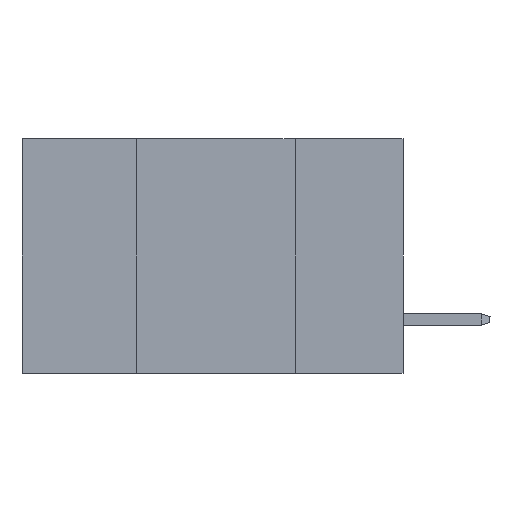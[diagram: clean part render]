
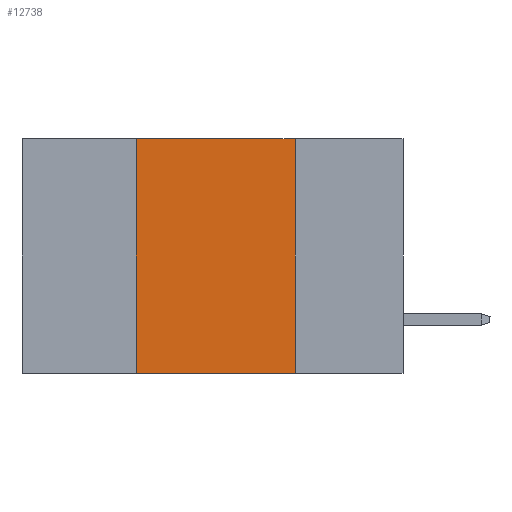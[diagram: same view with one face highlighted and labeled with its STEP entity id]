
A CAD part, left-side view. The second image highlights one B-rep face of the part: STEP entity #12738.
In plain terms, the highlighted planar face has unit normal (-1, 0, 0).
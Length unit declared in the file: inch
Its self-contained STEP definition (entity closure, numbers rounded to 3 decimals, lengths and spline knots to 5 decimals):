
#329 = CARTESIAN_POINT ( 'NONE',  ( 0., 0.17, 0. ) ) ;
#506 = DIRECTION ( 'NONE',  ( 0., -1., 0. ) ) ;
#595 = LINE ( 'NONE', #23482, #30440 ) ;
#2556 = DIRECTION ( 'NONE',  ( 0., 0., -1. ) ) ;
#3785 = ORIENTED_EDGE ( 'NONE', *, *, #19312, .F. ) ;
#4529 = VECTOR ( 'NONE', #7915, 39.37008 ) ;
#6155 = VECTOR ( 'NONE', #2556, 39.37008 ) ;
#6586 = VERTEX_POINT ( 'NONE', #329 ) ;
#7106 = DIRECTION ( 'NONE',  ( 0., 0., -1. ) ) ;
#7584 = EDGE_CURVE ( 'NONE', #13231, #32620, #595, .T. ) ;
#7915 = DIRECTION ( 'NONE',  ( 0., -1., 0. ) ) ;
#9631 = PLANE ( 'NONE',  #14361 ) ;
#10714 = CARTESIAN_POINT ( 'NONE',  ( 0., 0.6, 0. ) ) ;
#12442 = LINE ( 'NONE', #32649, #6155 ) ;
#12704 = CARTESIAN_POINT ( 'NONE',  ( 0., 0.17, -0.37 ) ) ;
#12738 = ADVANCED_FACE ( 'NONE', ( #32313 ), #9631, .F. ) ;
#13231 = VERTEX_POINT ( 'NONE', #21793 ) ;
#14119 = CARTESIAN_POINT ( 'NONE',  ( 0., 0.6, 0. ) ) ;
#14361 = AXIS2_PLACEMENT_3D ( 'NONE', #14119, #21833, #7106 ) ;
#15425 = ORIENTED_EDGE ( 'NONE', *, *, #17757, .T. ) ;
#15555 = LINE ( 'NONE', #10714, #30569 ) ;
#15640 = VERTEX_POINT ( 'NONE', #12704 ) ;
#16596 = EDGE_LOOP ( 'NONE', ( #3785, #28138, #16806, #15425 ) ) ;
#16806 = ORIENTED_EDGE ( 'NONE', *, *, #7584, .F. ) ;
#17757 = EDGE_CURVE ( 'NONE', #13231, #15640, #23117, .T. ) ;
#19312 = EDGE_CURVE ( 'NONE', #6586, #15640, #12442, .T. ) ;
#21793 = CARTESIAN_POINT ( 'NONE',  ( 0., 0.42, -0.37 ) ) ;
#21833 = DIRECTION ( 'NONE',  ( 1., 0., 0. ) ) ;
#23117 = LINE ( 'NONE', #30795, #4529 ) ;
#23482 = CARTESIAN_POINT ( 'NONE',  ( 0., 0.42, 0. ) ) ;
#23952 = CARTESIAN_POINT ( 'NONE',  ( 0., 0.42, 0. ) ) ;
#28138 = ORIENTED_EDGE ( 'NONE', *, *, #30180, .F. ) ;
#30180 = EDGE_CURVE ( 'NONE', #32620, #6586, #15555, .T. ) ;
#30440 = VECTOR ( 'NONE', #31169, 39.37008 ) ;
#30569 = VECTOR ( 'NONE', #506, 39.37008 ) ;
#30795 = CARTESIAN_POINT ( 'NONE',  ( 0., 0.6, -0.37 ) ) ;
#31169 = DIRECTION ( 'NONE',  ( 0., 0., 1. ) ) ;
#32313 = FACE_OUTER_BOUND ( 'NONE', #16596, .T. ) ;
#32620 = VERTEX_POINT ( 'NONE', #23952 ) ;
#32649 = CARTESIAN_POINT ( 'NONE',  ( 0., 0.17, 0. ) ) ;
